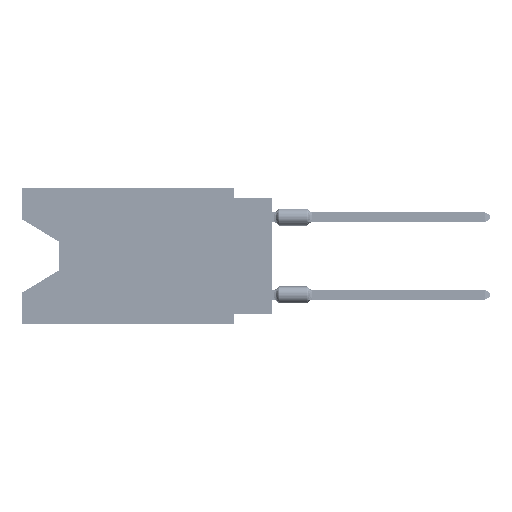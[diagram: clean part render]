
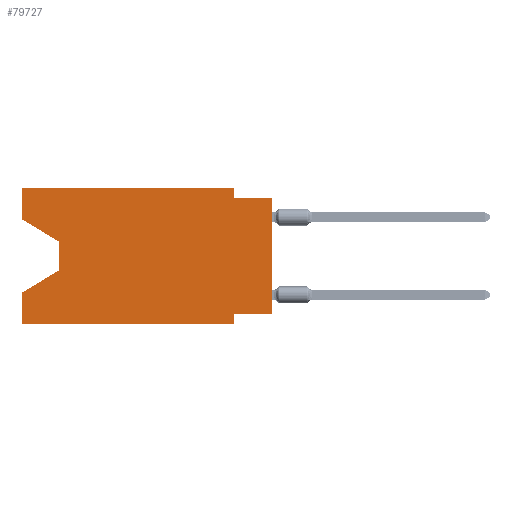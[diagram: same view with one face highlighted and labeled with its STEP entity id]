
A CAD part, left-side view. The second image highlights one B-rep face of the part: STEP entity #79727.
In plain terms, the highlighted planar face has unit normal (-1, 0, 0).
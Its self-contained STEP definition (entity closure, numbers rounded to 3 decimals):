
#108 = CARTESIAN_POINT ( 'NONE',  ( 0., 16.383, 0. ) ) ;
#249 = ORIENTED_EDGE ( 'NONE', *, *, #15101, .F. ) ;
#298 = VECTOR ( 'NONE', #79830, 1000. ) ;
#1259 = DIRECTION ( 'NONE',  ( 0., 1., 0. ) ) ;
#4175 = CARTESIAN_POINT ( 'NONE',  ( 0., 0., -8.255 ) ) ;
#4798 = ORIENTED_EDGE ( 'NONE', *, *, #63141, .T. ) ;
#4825 = ORIENTED_EDGE ( 'NONE', *, *, #19735, .F. ) ;
#5321 = CARTESIAN_POINT ( 'NONE',  ( 0., 16.383, 0. ) ) ;
#6586 = EDGE_CURVE ( 'NONE', #67910, #52068, #25347, .T. ) ;
#7345 = VECTOR ( 'NONE', #46239, 1000. ) ;
#7808 = CARTESIAN_POINT ( 'NONE',  ( 0., 0., -8.255 ) ) ;
#9472 = DIRECTION ( 'NONE',  ( 0., 0., -1. ) ) ;
#9654 = ORIENTED_EDGE ( 'NONE', *, *, #15927, .T. ) ;
#10134 = DIRECTION ( 'NONE',  ( 0., -0.855, -0.519 ) ) ;
#12068 = LINE ( 'NONE', #7808, #44645 ) ;
#13036 = LINE ( 'NONE', #41523, #17506 ) ;
#13352 = LINE ( 'NONE', #69446, #59420 ) ;
#14641 = DIRECTION ( 'NONE',  ( 0., -1., 0. ) ) ;
#15101 = EDGE_CURVE ( 'NONE', #91064, #67578, #91271, .T. ) ;
#15362 = PLANE ( 'NONE',  #30376 ) ;
#15902 = CARTESIAN_POINT ( 'NONE',  ( 0., 13.97, -5.385 ) ) ;
#15927 = EDGE_CURVE ( 'NONE', #92056, #54354, #13036, .T. ) ;
#17506 = VECTOR ( 'NONE', #44726, 1000. ) ;
#19735 = EDGE_CURVE ( 'NONE', #92056, #69959, #13352, .T. ) ;
#20125 = VERTEX_POINT ( 'NONE', #83791 ) ;
#21929 = DIRECTION ( 'NONE',  ( 0., 0., -1. ) ) ;
#21944 = CARTESIAN_POINT ( 'NONE',  ( 0., 0., -0.635 ) ) ;
#23050 = EDGE_CURVE ( 'NONE', #20125, #49603, #53700, .T. ) ;
#24814 = ORIENTED_EDGE ( 'NONE', *, *, #75574, .F. ) ;
#25347 = LINE ( 'NONE', #60903, #53340 ) ;
#27279 = ORIENTED_EDGE ( 'NONE', *, *, #30829, .T. ) ;
#29825 = CARTESIAN_POINT ( 'NONE',  ( 0., 16.383, 0. ) ) ;
#30376 = AXIS2_PLACEMENT_3D ( 'NONE', #29825, #35927, #21929 ) ;
#30829 = EDGE_CURVE ( 'NONE', #32828, #67910, #59646, .T. ) ;
#32828 = VERTEX_POINT ( 'NONE', #69091 ) ;
#33820 = DIRECTION ( 'NONE',  ( 0., 0., 1. ) ) ;
#33910 = VECTOR ( 'NONE', #9472, 1000. ) ;
#34442 = VERTEX_POINT ( 'NONE', #4175 ) ;
#35927 = DIRECTION ( 'NONE',  ( 1., 0., 0. ) ) ;
#38016 = CARTESIAN_POINT ( 'NONE',  ( 0., 2.54, -8.89 ) ) ;
#38779 = ORIENTED_EDGE ( 'NONE', *, *, #23050, .F. ) ;
#41021 = VECTOR ( 'NONE', #10134, 1000. ) ;
#41523 = CARTESIAN_POINT ( 'NONE',  ( 0., 16.383, -8.89 ) ) ;
#44141 = CARTESIAN_POINT ( 'NONE',  ( 0., 2.54, 0. ) ) ;
#44566 = ORIENTED_EDGE ( 'NONE', *, *, #78531, .T. ) ;
#44645 = VECTOR ( 'NONE', #1259, 1000. ) ;
#44726 = DIRECTION ( 'NONE',  ( 0., -1., 0. ) ) ;
#44945 = ORIENTED_EDGE ( 'NONE', *, *, #69249, .F. ) ;
#46239 = DIRECTION ( 'NONE',  ( 0., -1., 0. ) ) ;
#49603 = VERTEX_POINT ( 'NONE', #21944 ) ;
#51107 = LINE ( 'NONE', #38016, #85639 ) ;
#52068 = VERTEX_POINT ( 'NONE', #80179 ) ;
#52626 = CARTESIAN_POINT ( 'NONE',  ( 0., 16.383, -2.038 ) ) ;
#52954 = DIRECTION ( 'NONE',  ( 0., 0., -1. ) ) ;
#53340 = VECTOR ( 'NONE', #52954, 1000. ) ;
#53689 = EDGE_CURVE ( 'NONE', #78339, #54354, #51107, .T. ) ;
#53700 = LINE ( 'NONE', #75207, #7345 ) ;
#54354 = VERTEX_POINT ( 'NONE', #70908 ) ;
#54707 = ORIENTED_EDGE ( 'NONE', *, *, #61540, .F. ) ;
#55312 = LINE ( 'NONE', #5321, #91182 ) ;
#58090 = CARTESIAN_POINT ( 'NONE',  ( 0., 2.54, 0. ) ) ;
#58323 = EDGE_LOOP ( 'NONE', ( #27279, #59102, #4798, #4825, #9654, #83316, #54707, #44566, #38779, #44945, #249, #24814 ) ) ;
#59102 = ORIENTED_EDGE ( 'NONE', *, *, #6586, .T. ) ;
#59420 = VECTOR ( 'NONE', #70815, 1000. ) ;
#59646 = LINE ( 'NONE', #52626, #41021 ) ;
#60903 = CARTESIAN_POINT ( 'NONE',  ( 0., 13.97, -3.505 ) ) ;
#61540 = EDGE_CURVE ( 'NONE', #34442, #78339, #12068, .T. ) ;
#63141 = EDGE_CURVE ( 'NONE', #52068, #69959, #79907, .T. ) ;
#64881 = CARTESIAN_POINT ( 'NONE',  ( 0., 0., 0. ) ) ;
#65803 = LINE ( 'NONE', #64881, #298 ) ;
#67578 = VERTEX_POINT ( 'NONE', #44141 ) ;
#67619 = VECTOR ( 'NONE', #73362, 1000. ) ;
#67910 = VERTEX_POINT ( 'NONE', #79538 ) ;
#69091 = CARTESIAN_POINT ( 'NONE',  ( 0., 16.383, -2.038 ) ) ;
#69249 = EDGE_CURVE ( 'NONE', #67578, #20125, #80492, .T. ) ;
#69446 = CARTESIAN_POINT ( 'NONE',  ( 0., 16.383, 0. ) ) ;
#69959 = VERTEX_POINT ( 'NONE', #84040 ) ;
#70815 = DIRECTION ( 'NONE',  ( 0., 0., 1. ) ) ;
#70908 = CARTESIAN_POINT ( 'NONE',  ( 0., 2.54, -8.89 ) ) ;
#71904 = CARTESIAN_POINT ( 'NONE',  ( 0., 16.383, 0. ) ) ;
#72721 = CARTESIAN_POINT ( 'NONE',  ( 0., 2.54, -8.255 ) ) ;
#73301 = FACE_OUTER_BOUND ( 'NONE', #58323, .T. ) ;
#73362 = DIRECTION ( 'NONE',  ( 0., 0.855, -0.519 ) ) ;
#75207 = CARTESIAN_POINT ( 'NONE',  ( 0., 0., -0.635 ) ) ;
#75574 = EDGE_CURVE ( 'NONE', #32828, #91064, #55312, .T. ) ;
#78339 = VERTEX_POINT ( 'NONE', #72721 ) ;
#78531 = EDGE_CURVE ( 'NONE', #34442, #49603, #65803, .T. ) ;
#79538 = CARTESIAN_POINT ( 'NONE',  ( 0., 13.97, -3.505 ) ) ;
#79727 = ADVANCED_FACE ( 'NONE', ( #73301 ), #15362, .F. ) ;
#79830 = DIRECTION ( 'NONE',  ( 0., 0., 1. ) ) ;
#79907 = LINE ( 'NONE', #15902, #67619 ) ;
#80179 = CARTESIAN_POINT ( 'NONE',  ( 0., 13.97, -5.385 ) ) ;
#80492 = LINE ( 'NONE', #58090, #33910 ) ;
#80544 = DIRECTION ( 'NONE',  ( 0., 0., -1. ) ) ;
#83040 = VECTOR ( 'NONE', #14641, 1000. ) ;
#83316 = ORIENTED_EDGE ( 'NONE', *, *, #53689, .F. ) ;
#83791 = CARTESIAN_POINT ( 'NONE',  ( 0., 2.54, -0.635 ) ) ;
#84040 = CARTESIAN_POINT ( 'NONE',  ( 0., 16.383, -6.852 ) ) ;
#85118 = CARTESIAN_POINT ( 'NONE',  ( 0., 16.383, -8.89 ) ) ;
#85639 = VECTOR ( 'NONE', #80544, 1000. ) ;
#91064 = VERTEX_POINT ( 'NONE', #71904 ) ;
#91182 = VECTOR ( 'NONE', #33820, 1000. ) ;
#91271 = LINE ( 'NONE', #108, #83040 ) ;
#92056 = VERTEX_POINT ( 'NONE', #85118 ) ;
